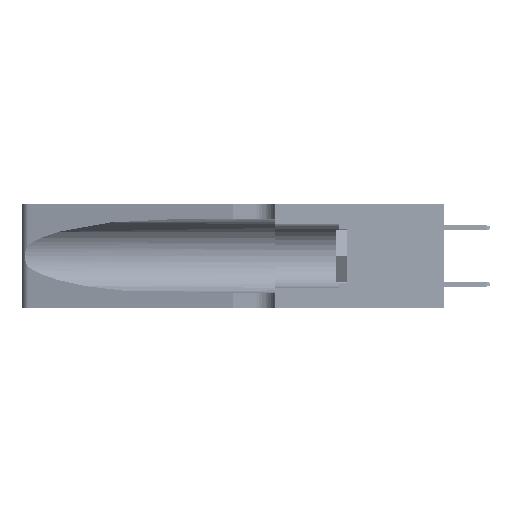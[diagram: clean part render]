
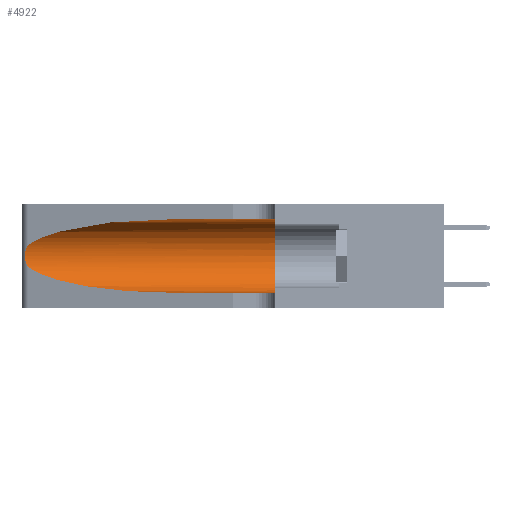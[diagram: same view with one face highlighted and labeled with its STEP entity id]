
A CAD part, left-side view. The second image highlights one B-rep face of the part: STEP entity #4922.
In plain terms, the highlighted cylindrical face has radius 3.308 mm (diameter 6.617 mm), a partial arc.
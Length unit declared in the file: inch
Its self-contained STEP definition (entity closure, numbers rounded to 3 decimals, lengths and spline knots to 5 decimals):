
#137 = CARTESIAN_POINT ( 'NONE',  ( 0.25487, 1.22718, 0.14631 ) ) ;
#879 = EDGE_CURVE ( 'NONE', #12759, #14028, #38346, .T. ) ;
#1617 = CARTESIAN_POINT ( 'NONE',  ( 0.1305, 0.72297, 0.05475 ) ) ;
#2094 = DIRECTION ( 'NONE',  ( 0., 1., 0. ) ) ;
#3186 = CARTESIAN_POINT ( 'NONE',  ( 0.25487, 1.22718, 0.14631 ) ) ;
#3410 = CARTESIAN_POINT ( 'NONE',  ( 0.25487, 1.22718, 0.22369 ) ) ;
#4109 = CARTESIAN_POINT ( 'NONE',  ( 0.18966, 0.96281, 0.31525 ) ) ;
#4226 = LINE ( 'NONE', #27679, #45216 ) ;
#4847 = DIRECTION ( 'NONE',  ( 0., -1., 0. ) ) ;
#4922 = ADVANCED_FACE ( 'NONE', ( #30670 ), #23796, .F. ) ;
#5099 = EDGE_CURVE ( 'NONE', #14028, #17340, #41196, .T. ) ;
#5326 = AXIS2_PLACEMENT_3D ( 'NONE', #17533, #2094, #34578 ) ;
#8405 = B_SPLINE_CURVE_WITH_KNOTS ( 'NONE', 3,
 ( #48578, #49266, #28623, #25107, #37130, #8839, #37314, #13497, #33130, #32611, #40778, #16948, #12798, #9325 ),
 .UNSPECIFIED., .F., .F.,
 ( 4, 2, 2, 2, 2, 2, 4 ),
 ( 0., 0.00027, 0.00053, 0.00107, 0.0016, 0.00187, 0.00214 ),
 .UNSPECIFIED. ) ;
#8719 = EDGE_LOOP ( 'NONE', ( #32543, #26657, #39078, #28616, #30656, #28442 ) ) ;
#8839 = CARTESIAN_POINT ( 'NONE',  ( 0.26018, 1.23835, 0.19895 ) ) ;
#9325 = CARTESIAN_POINT ( 'NONE',  ( 0.25487, 1.22718, 0.14631 ) ) ;
#10798 = VERTEX_POINT ( 'NONE', #32817 ) ;
#10799 = CARTESIAN_POINT ( 'NONE',  ( 0.1305, 0.35, 0.31525 ) ) ;
#12366 = EDGE_CURVE ( 'NONE', #22181, #17340, #13642, .T. ) ;
#12759 = VERTEX_POINT ( 'NONE', #137 ) ;
#12798 = CARTESIAN_POINT ( 'NONE',  ( 0.25555, 1.22993, 0.14849 ) ) ;
#12811 = CARTESIAN_POINT ( 'NONE',  ( 0.1305, 1.61858, 0.185 ) ) ;
#13497 = CARTESIAN_POINT ( 'NONE',  ( 0.26075, 1.23896, 0.178 ) ) ;
#13642 = CIRCLE ( 'NONE', #5326, 0.13025 ) ;
#13826 = VECTOR ( 'NONE', #36803, 39.37008 ) ;
#14028 = VERTEX_POINT ( 'NONE', #1617 ) ;
#16948 = CARTESIAN_POINT ( 'NONE',  ( 0.25639, 1.23186, 0.15144 ) ) ;
#17340 = VERTEX_POINT ( 'NONE', #21097 ) ;
#17533 = CARTESIAN_POINT ( 'NONE',  ( 0.1305, 0.35, 0.185 ) ) ;
#18952 = CARTESIAN_POINT ( 'NONE',  ( 0.2373, 1.15595, 0.08982 ) ) ;
#19684 = EDGE_CURVE ( 'NONE', #29866, #10798, #45317, .T. ) ;
#21097 = CARTESIAN_POINT ( 'NONE',  ( 0.1305, 0.35, 0.05475 ) ) ;
#22181 = VERTEX_POINT ( 'NONE', #10799 ) ;
#23475 = DIRECTION ( 'NONE',  ( 0., -1., 0. ) ) ;
#23796 = CYLINDRICAL_SURFACE ( 'NONE', #43741, 0.13025 ) ;
#25107 = CARTESIAN_POINT ( 'NONE',  ( 0.25787, 1.23484, 0.2124 ) ) ;
#26657 = ORIENTED_EDGE ( 'NONE', *, *, #35726, .T. ) ;
#27545 = EDGE_CURVE ( 'NONE', #29866, #22181, #4226, .T. ) ;
#27679 = CARTESIAN_POINT ( 'NONE',  ( 0.1305, 1.61858, 0.31525 ) ) ;
#28442 = ORIENTED_EDGE ( 'NONE', *, *, #27545, .F. ) ;
#28616 = ORIENTED_EDGE ( 'NONE', *, *, #5099, .T. ) ;
#28623 = CARTESIAN_POINT ( 'NONE',  ( 0.25639, 1.23184, 0.21858 ) ) ;
#29866 = VERTEX_POINT ( 'NONE', #46921 ) ;
#30656 = ORIENTED_EDGE ( 'NONE', *, *, #12366, .F. ) ;
#30670 = FACE_OUTER_BOUND ( 'NONE', #8719, .T. ) ;
#32300 = DIRECTION ( 'NONE',  ( 0., 0., -1. ) ) ;
#32543 = ORIENTED_EDGE ( 'NONE', *, *, #19684, .T. ) ;
#32611 = CARTESIAN_POINT ( 'NONE',  ( 0.25856, 1.23593, 0.16098 ) ) ;
#32817 = CARTESIAN_POINT ( 'NONE',  ( 0.25487, 1.22718, 0.22369 ) ) ;
#33130 = CARTESIAN_POINT ( 'NONE',  ( 0.26017, 1.23833, 0.17102 ) ) ;
#34578 = DIRECTION ( 'NONE',  ( 0., 0., 1. ) ) ;
#35364 = CARTESIAN_POINT ( 'NONE',  ( 0.1305, 0.72297, 0.31525 ) ) ;
#35726 = EDGE_CURVE ( 'NONE', #10798, #12759, #8405, .T. ) ;
#36803 = DIRECTION ( 'NONE',  ( 0., -1., 0. ) ) ;
#37130 = CARTESIAN_POINT ( 'NONE',  ( 0.25854, 1.2359, 0.20912 ) ) ;
#37314 = CARTESIAN_POINT ( 'NONE',  ( 0.26075, 1.23896, 0.19203 ) ) ;
#37327 = CARTESIAN_POINT ( 'NONE',  ( 0.1305, 1.61858, 0.05475 ) ) ;
#38346 =( BOUNDED_CURVE ( )  B_SPLINE_CURVE ( 3, ( #3186, #18952, #42963, #39144 ),
 .UNSPECIFIED., .F., .F. ) 
 B_SPLINE_CURVE_WITH_KNOTS ( ( 4, 4 ),
 ( 3.44316, 4.71239 ),
 .UNSPECIFIED. ) 
 CURVE ( )  GEOMETRIC_REPRESENTATION_ITEM ( )  RATIONAL_B_SPLINE_CURVE ( ( 1., 0.87, 0.87, 1. ) ) 
 REPRESENTATION_ITEM ( '' )  );
#39078 = ORIENTED_EDGE ( 'NONE', *, *, #879, .T. ) ;
#39144 = CARTESIAN_POINT ( 'NONE',  ( 0.1305, 0.72297, 0.05475 ) ) ;
#39365 = CARTESIAN_POINT ( 'NONE',  ( 0.2373, 1.15595, 0.28018 ) ) ;
#40778 = CARTESIAN_POINT ( 'NONE',  ( 0.25789, 1.23486, 0.15765 ) ) ;
#41196 = LINE ( 'NONE', #37327, #13826 ) ;
#42963 = CARTESIAN_POINT ( 'NONE',  ( 0.18966, 0.96281, 0.05475 ) ) ;
#43741 = AXIS2_PLACEMENT_3D ( 'NONE', #12811, #4847, #32300 ) ;
#45216 = VECTOR ( 'NONE', #23475, 39.37008 ) ;
#45317 =( BOUNDED_CURVE ( )  B_SPLINE_CURVE ( 3, ( #35364, #4109, #39365, #3410 ),
 .UNSPECIFIED., .F., .F. ) 
 B_SPLINE_CURVE_WITH_KNOTS ( ( 4, 4 ),
 ( 1.5708, 2.84003 ),
 .UNSPECIFIED. ) 
 CURVE ( )  GEOMETRIC_REPRESENTATION_ITEM ( )  RATIONAL_B_SPLINE_CURVE ( ( 1., 0.87, 0.87, 1. ) ) 
 REPRESENTATION_ITEM ( '' )  );
#46921 = CARTESIAN_POINT ( 'NONE',  ( 0.1305, 0.72297, 0.31525 ) ) ;
#48578 = CARTESIAN_POINT ( 'NONE',  ( 0.25487, 1.22718, 0.22369 ) ) ;
#49266 = CARTESIAN_POINT ( 'NONE',  ( 0.25555, 1.22994, 0.2215 ) ) ;
